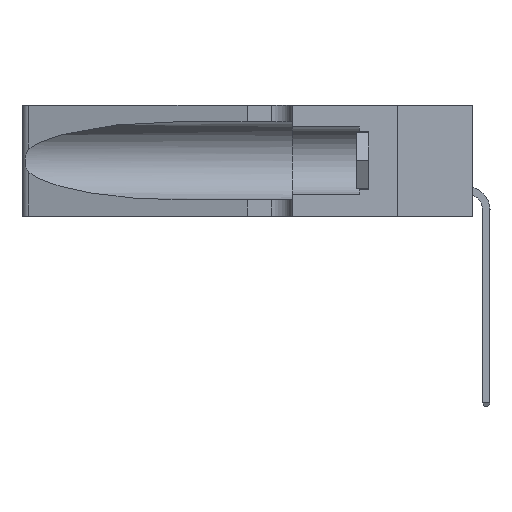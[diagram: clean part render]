
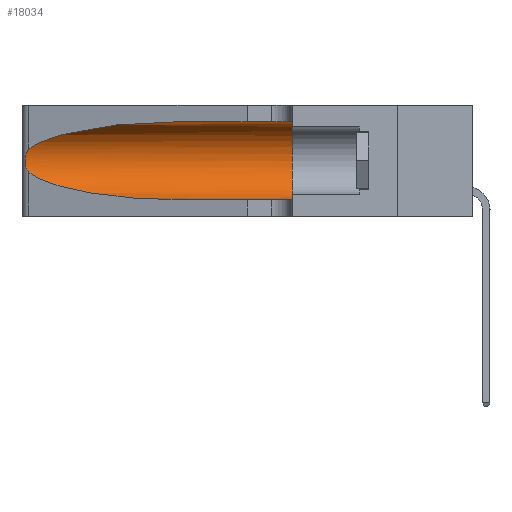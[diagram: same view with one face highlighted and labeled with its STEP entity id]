
A CAD part, left-side view. The second image highlights one B-rep face of the part: STEP entity #18034.
In plain terms, the highlighted cylindrical face has radius 3.308 mm (diameter 6.617 mm), a partial arc.
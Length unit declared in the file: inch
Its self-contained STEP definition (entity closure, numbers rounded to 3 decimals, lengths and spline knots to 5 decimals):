
#16 = CARTESIAN_POINT ( 'NONE',  ( 0.2373, 1.15595, 0.08982 ) ) ;
#165 = DIRECTION ( 'NONE',  ( 0., -1., 0. ) ) ;
#621 = CARTESIAN_POINT ( 'NONE',  ( 0.1305, 0.72297, 0.31525 ) ) ;
#725 = CARTESIAN_POINT ( 'NONE',  ( 0.25487, 1.22718, 0.22369 ) ) ;
#898 = CARTESIAN_POINT ( 'NONE',  ( 0.26017, 1.23833, 0.17102 ) ) ;
#2033 = CARTESIAN_POINT ( 'NONE',  ( 0.1305, 1.61858, 0.185 ) ) ;
#2088 = ORIENTED_EDGE ( 'NONE', *, *, #2749, .T. ) ;
#2432 = CARTESIAN_POINT ( 'NONE',  ( 0.25639, 1.23184, 0.21858 ) ) ;
#2452 = CYLINDRICAL_SURFACE ( 'NONE', #22945, 0.13025 ) ;
#2749 = EDGE_CURVE ( 'NONE', #23273, #15920, #21789, .T. ) ;
#3612 = VERTEX_POINT ( 'NONE', #23009 ) ;
#4119 = DIRECTION ( 'NONE',  ( 0., 1., 0. ) ) ;
#4286 = CARTESIAN_POINT ( 'NONE',  ( 0.26075, 1.23896, 0.19203 ) ) ;
#4445 = CARTESIAN_POINT ( 'NONE',  ( 0.26018, 1.23835, 0.19895 ) ) ;
#4767 = VECTOR ( 'NONE', #13692, 39.37008 ) ;
#5068 = DIRECTION ( 'NONE',  ( 0., -1., 0. ) ) ;
#5368 = CARTESIAN_POINT ( 'NONE',  ( 0.1305, 0.72297, 0.31525 ) ) ;
#5411 = CARTESIAN_POINT ( 'NONE',  ( 0.25487, 1.22718, 0.22369 ) ) ;
#5596 = DIRECTION ( 'NONE',  ( 0., 0., -1. ) ) ;
#5665 = B_SPLINE_CURVE_WITH_KNOTS ( 'NONE', 3,
 ( #725, #17245, #2432, #15382, #8213, #4445, #4286, #21193, #898, #6146, #19103, #23056, #20964, #9921 ),
 .UNSPECIFIED., .F., .F.,
 ( 4, 2, 2, 2, 2, 2, 4 ),
 ( 0., 0.00027, 0.00053, 0.00107, 0.0016, 0.00187, 0.00214 ),
 .UNSPECIFIED. ) ;
#5877 = EDGE_CURVE ( 'NONE', #20899, #23273, #13549, .T. ) ;
#6146 = CARTESIAN_POINT ( 'NONE',  ( 0.25856, 1.23593, 0.16098 ) ) ;
#6391 = ORIENTED_EDGE ( 'NONE', *, *, #5877, .T. ) ;
#7968 = ORIENTED_EDGE ( 'NONE', *, *, #13601, .F. ) ;
#8153 = VECTOR ( 'NONE', #5068, 39.37008 ) ;
#8213 = CARTESIAN_POINT ( 'NONE',  ( 0.25854, 1.2359, 0.20912 ) ) ;
#9239 = CARTESIAN_POINT ( 'NONE',  ( 0.25487, 1.22718, 0.14631 ) ) ;
#9294 = CARTESIAN_POINT ( 'NONE',  ( 0.1305, 0.72297, 0.05475 ) ) ;
#9663 = LINE ( 'NONE', #17333, #4767 ) ;
#9921 = CARTESIAN_POINT ( 'NONE',  ( 0.25487, 1.22718, 0.14631 ) ) ;
#11342 = EDGE_CURVE ( 'NONE', #18586, #20899, #5665, .T. ) ;
#12370 = EDGE_CURVE ( 'NONE', #17754, #18586, #23179, .T. ) ;
#13140 = AXIS2_PLACEMENT_3D ( 'NONE', #13613, #4119, #20966 ) ;
#13452 = ORIENTED_EDGE ( 'NONE', *, *, #11342, .T. ) ;
#13546 = EDGE_CURVE ( 'NONE', #3612, #15920, #15487, .T. ) ;
#13549 =( BOUNDED_CURVE ( )  B_SPLINE_CURVE ( 3, ( #16773, #16, #18711, #9294 ),
 .UNSPECIFIED., .F., .F. ) 
 B_SPLINE_CURVE_WITH_KNOTS ( ( 4, 4 ),
 ( 3.44316, 4.71239 ),
 .UNSPECIFIED. ) 
 CURVE ( )  GEOMETRIC_REPRESENTATION_ITEM ( )  RATIONAL_B_SPLINE_CURVE ( ( 1., 0.87, 0.87, 1. ) ) 
 REPRESENTATION_ITEM ( '' )  );
#13601 = EDGE_CURVE ( 'NONE', #17754, #3612, #9663, .T. ) ;
#13613 = CARTESIAN_POINT ( 'NONE',  ( 0.1305, 0.35, 0.185 ) ) ;
#13692 = DIRECTION ( 'NONE',  ( 0., -1., 0. ) ) ;
#14394 = CARTESIAN_POINT ( 'NONE',  ( 0.1305, 1.61858, 0.05475 ) ) ;
#15382 = CARTESIAN_POINT ( 'NONE',  ( 0.25787, 1.23484, 0.2124 ) ) ;
#15487 = CIRCLE ( 'NONE', #13140, 0.13025 ) ;
#15744 = ORIENTED_EDGE ( 'NONE', *, *, #13546, .F. ) ;
#15920 = VERTEX_POINT ( 'NONE', #23906 ) ;
#16160 = EDGE_LOOP ( 'NONE', ( #17378, #13452, #6391, #2088, #15744, #7968 ) ) ;
#16773 = CARTESIAN_POINT ( 'NONE',  ( 0.25487, 1.22718, 0.14631 ) ) ;
#17245 = CARTESIAN_POINT ( 'NONE',  ( 0.25555, 1.22994, 0.2215 ) ) ;
#17310 = CARTESIAN_POINT ( 'NONE',  ( 0.2373, 1.15595, 0.28018 ) ) ;
#17333 = CARTESIAN_POINT ( 'NONE',  ( 0.1305, 1.61858, 0.31525 ) ) ;
#17378 = ORIENTED_EDGE ( 'NONE', *, *, #12370, .T. ) ;
#17383 = CARTESIAN_POINT ( 'NONE',  ( 0.18966, 0.96281, 0.31525 ) ) ;
#17754 = VERTEX_POINT ( 'NONE', #5368 ) ;
#18034 = ADVANCED_FACE ( 'NONE', ( #20403 ), #2452, .F. ) ;
#18534 = CARTESIAN_POINT ( 'NONE',  ( 0.1305, 0.72297, 0.05475 ) ) ;
#18586 = VERTEX_POINT ( 'NONE', #5411 ) ;
#18711 = CARTESIAN_POINT ( 'NONE',  ( 0.18966, 0.96281, 0.05475 ) ) ;
#19103 = CARTESIAN_POINT ( 'NONE',  ( 0.25789, 1.23486, 0.15765 ) ) ;
#20403 = FACE_OUTER_BOUND ( 'NONE', #16160, .T. ) ;
#20899 = VERTEX_POINT ( 'NONE', #9239 ) ;
#20964 = CARTESIAN_POINT ( 'NONE',  ( 0.25555, 1.22993, 0.14849 ) ) ;
#20966 = DIRECTION ( 'NONE',  ( 0., 0., 1. ) ) ;
#21172 = CARTESIAN_POINT ( 'NONE',  ( 0.25487, 1.22718, 0.22369 ) ) ;
#21193 = CARTESIAN_POINT ( 'NONE',  ( 0.26075, 1.23896, 0.178 ) ) ;
#21789 = LINE ( 'NONE', #14394, #8153 ) ;
#22945 = AXIS2_PLACEMENT_3D ( 'NONE', #2033, #165, #5596 ) ;
#23009 = CARTESIAN_POINT ( 'NONE',  ( 0.1305, 0.35, 0.31525 ) ) ;
#23056 = CARTESIAN_POINT ( 'NONE',  ( 0.25639, 1.23186, 0.15144 ) ) ;
#23179 =( BOUNDED_CURVE ( )  B_SPLINE_CURVE ( 3, ( #621, #17383, #17310, #21172 ),
 .UNSPECIFIED., .F., .F. ) 
 B_SPLINE_CURVE_WITH_KNOTS ( ( 4, 4 ),
 ( 1.5708, 2.84003 ),
 .UNSPECIFIED. ) 
 CURVE ( )  GEOMETRIC_REPRESENTATION_ITEM ( )  RATIONAL_B_SPLINE_CURVE ( ( 1., 0.87, 0.87, 1. ) ) 
 REPRESENTATION_ITEM ( '' )  );
#23273 = VERTEX_POINT ( 'NONE', #18534 ) ;
#23906 = CARTESIAN_POINT ( 'NONE',  ( 0.1305, 0.35, 0.05475 ) ) ;
